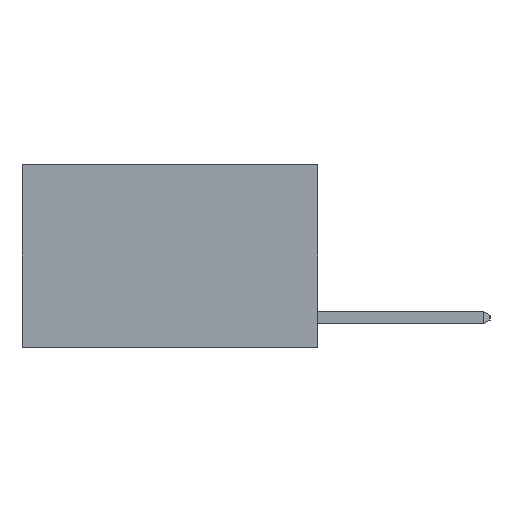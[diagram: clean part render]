
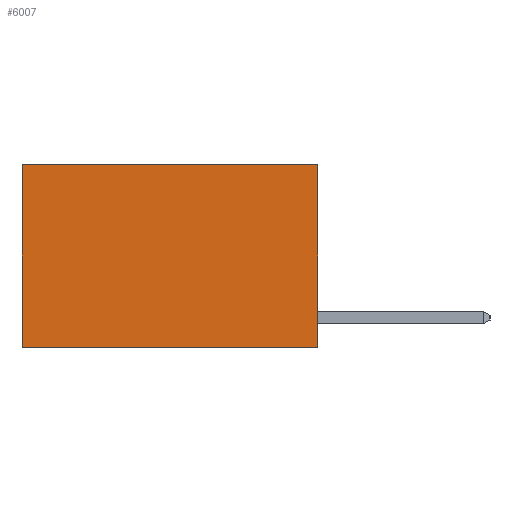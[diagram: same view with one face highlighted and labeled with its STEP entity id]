
A CAD part, left-side view. The second image highlights one B-rep face of the part: STEP entity #6007.
In plain terms, the highlighted planar face has unit normal (-1, 0, 0).
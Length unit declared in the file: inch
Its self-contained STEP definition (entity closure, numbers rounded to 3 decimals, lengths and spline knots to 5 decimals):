
#208 = EDGE_CURVE ( 'NONE', #5028, #7236, #3110, .T. ) ;
#631 = CARTESIAN_POINT ( 'NONE',  ( 0.2625, 0., 0. ) ) ;
#733 = CARTESIAN_POINT ( 'NONE',  ( 0.2625, 0.6, -0.37 ) ) ;
#1376 = CARTESIAN_POINT ( 'NONE',  ( 0.2625, 0., 0. ) ) ;
#1533 = LINE ( 'NONE', #4720, #3032 ) ;
#2038 = DIRECTION ( 'NONE',  ( 0., 0., -1. ) ) ;
#2170 = DIRECTION ( 'NONE',  ( 0., 0., -1. ) ) ;
#2344 = EDGE_CURVE ( 'NONE', #5522, #7236, #1533, .T. ) ;
#2401 = LINE ( 'NONE', #631, #5613 ) ;
#2548 = CARTESIAN_POINT ( 'NONE',  ( 0.2625, 0., -0.37 ) ) ;
#2844 = ORIENTED_EDGE ( 'NONE', *, *, #4302, .F. ) ;
#3032 = VECTOR ( 'NONE', #2170, 39.37008 ) ;
#3110 = LINE ( 'NONE', #2548, #6133 ) ;
#3194 = VECTOR ( 'NONE', #6315, 39.37008 ) ;
#3210 = DIRECTION ( 'NONE',  ( 0., 0., -1. ) ) ;
#4007 = CARTESIAN_POINT ( 'NONE',  ( 0.2625, 0., -0.37 ) ) ;
#4193 = EDGE_CURVE ( 'NONE', #7035, #5522, #6819, .T. ) ;
#4302 = EDGE_CURVE ( 'NONE', #7035, #5028, #2401, .T. ) ;
#4323 = EDGE_LOOP ( 'NONE', ( #6740, #6182, #2844, #6453 ) ) ;
#4568 = AXIS2_PLACEMENT_3D ( 'NONE', #1376, #5880, #2038 ) ;
#4720 = CARTESIAN_POINT ( 'NONE',  ( 0.2625, 0.6, 0. ) ) ;
#5028 = VERTEX_POINT ( 'NONE', #4007 ) ;
#5522 = VERTEX_POINT ( 'NONE', #5857 ) ;
#5613 = VECTOR ( 'NONE', #3210, 39.37008 ) ;
#5670 = CARTESIAN_POINT ( 'NONE',  ( 0.2625, 0., 0. ) ) ;
#5674 = CARTESIAN_POINT ( 'NONE',  ( 0.2625, 0., 0. ) ) ;
#5778 = DIRECTION ( 'NONE',  ( 0., 1., 0. ) ) ;
#5857 = CARTESIAN_POINT ( 'NONE',  ( 0.2625, 0.6, 0. ) ) ;
#5880 = DIRECTION ( 'NONE',  ( 1., 0., 0. ) ) ;
#6007 = ADVANCED_FACE ( 'NONE', ( #7570 ), #7769, .F. ) ;
#6133 = VECTOR ( 'NONE', #5778, 39.37008 ) ;
#6182 = ORIENTED_EDGE ( 'NONE', *, *, #208, .F. ) ;
#6315 = DIRECTION ( 'NONE',  ( 0., 1., 0. ) ) ;
#6453 = ORIENTED_EDGE ( 'NONE', *, *, #4193, .T. ) ;
#6740 = ORIENTED_EDGE ( 'NONE', *, *, #2344, .T. ) ;
#6819 = LINE ( 'NONE', #5674, #3194 ) ;
#7035 = VERTEX_POINT ( 'NONE', #5670 ) ;
#7236 = VERTEX_POINT ( 'NONE', #733 ) ;
#7570 = FACE_OUTER_BOUND ( 'NONE', #4323, .T. ) ;
#7769 = PLANE ( 'NONE',  #4568 ) ;
